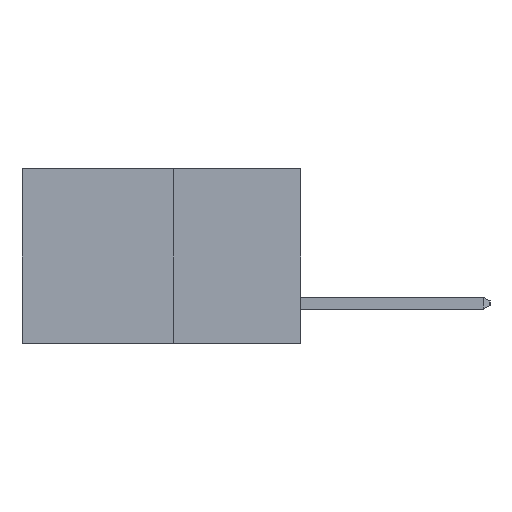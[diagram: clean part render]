
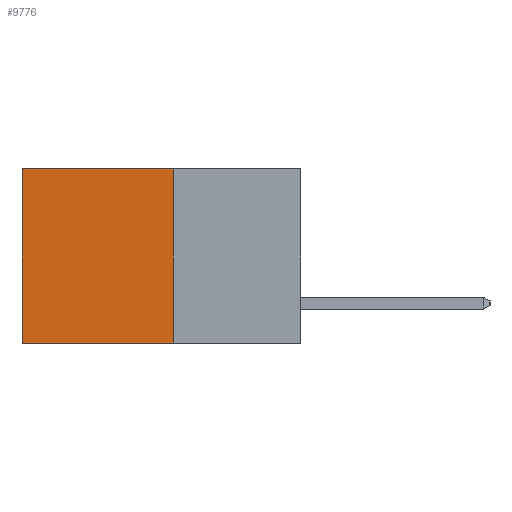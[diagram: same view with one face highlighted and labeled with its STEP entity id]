
A CAD part, left-side view. The second image highlights one B-rep face of the part: STEP entity #9776.
In plain terms, the highlighted planar face has unit normal (-1, 0, 0).
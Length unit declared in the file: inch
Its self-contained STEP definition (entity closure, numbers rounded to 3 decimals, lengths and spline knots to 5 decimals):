
#128 = VECTOR ( 'NONE', #5914, 39.37008 ) ;
#221 = DIRECTION ( 'NONE',  ( 0., 0., -1. ) ) ;
#391 = LINE ( 'NONE', #7999, #128 ) ;
#614 = LINE ( 'NONE', #7088, #4427 ) ;
#839 = PLANE ( 'NONE',  #6479 ) ;
#883 = CARTESIAN_POINT ( 'NONE',  ( 0.277, 0.59, 0. ) ) ;
#1371 = EDGE_CURVE ( 'NONE', #7778, #8145, #614, .T. ) ;
#1674 = DIRECTION ( 'NONE',  ( 1., 0., 0. ) ) ;
#1992 = CARTESIAN_POINT ( 'NONE',  ( 0.277, 0.27, -0.37 ) ) ;
#2012 = VECTOR ( 'NONE', #9882, 39.37008 ) ;
#2217 = ORIENTED_EDGE ( 'NONE', *, *, #1371, .T. ) ;
#2417 = EDGE_CURVE ( 'NONE', #3599, #8145, #7338, .T. ) ;
#2490 = ORIENTED_EDGE ( 'NONE', *, *, #6832, .F. ) ;
#2521 = EDGE_LOOP ( 'NONE', ( #2217, #3475, #2490, #5330 ) ) ;
#2647 = VERTEX_POINT ( 'NONE', #5793 ) ;
#2827 = EDGE_CURVE ( 'NONE', #2647, #7778, #391, .T. ) ;
#3183 = DIRECTION ( 'NONE',  ( 0., 1., 0. ) ) ;
#3252 = CARTESIAN_POINT ( 'NONE',  ( 0.277, 0.27, -0.37 ) ) ;
#3475 = ORIENTED_EDGE ( 'NONE', *, *, #2417, .F. ) ;
#3599 = VERTEX_POINT ( 'NONE', #1992 ) ;
#4134 = LINE ( 'NONE', #9836, #2012 ) ;
#4427 = VECTOR ( 'NONE', #221, 39.37008 ) ;
#4971 = VECTOR ( 'NONE', #3183, 39.37008 ) ;
#5330 = ORIENTED_EDGE ( 'NONE', *, *, #2827, .T. ) ;
#5793 = CARTESIAN_POINT ( 'NONE',  ( 0.277, 0.27, 0. ) ) ;
#5914 = DIRECTION ( 'NONE',  ( 0., 1., 0. ) ) ;
#6479 = AXIS2_PLACEMENT_3D ( 'NONE', #3252, #1674, #7238 ) ;
#6779 = CARTESIAN_POINT ( 'NONE',  ( 0.277, 0.27, -0.37 ) ) ;
#6818 = CARTESIAN_POINT ( 'NONE',  ( 0.277, 0.59, -0.37 ) ) ;
#6832 = EDGE_CURVE ( 'NONE', #2647, #3599, #4134, .T. ) ;
#7088 = CARTESIAN_POINT ( 'NONE',  ( 0.277, 0.59, -0.37 ) ) ;
#7238 = DIRECTION ( 'NONE',  ( 0., 0., -1. ) ) ;
#7338 = LINE ( 'NONE', #6779, #4971 ) ;
#7778 = VERTEX_POINT ( 'NONE', #883 ) ;
#7999 = CARTESIAN_POINT ( 'NONE',  ( 0.277, 0.27, 0. ) ) ;
#8145 = VERTEX_POINT ( 'NONE', #6818 ) ;
#9707 = FACE_OUTER_BOUND ( 'NONE', #2521, .T. ) ;
#9776 = ADVANCED_FACE ( 'NONE', ( #9707 ), #839, .F. ) ;
#9836 = CARTESIAN_POINT ( 'NONE',  ( 0.277, 0.27, -0.37 ) ) ;
#9882 = DIRECTION ( 'NONE',  ( 0., 0., -1. ) ) ;
